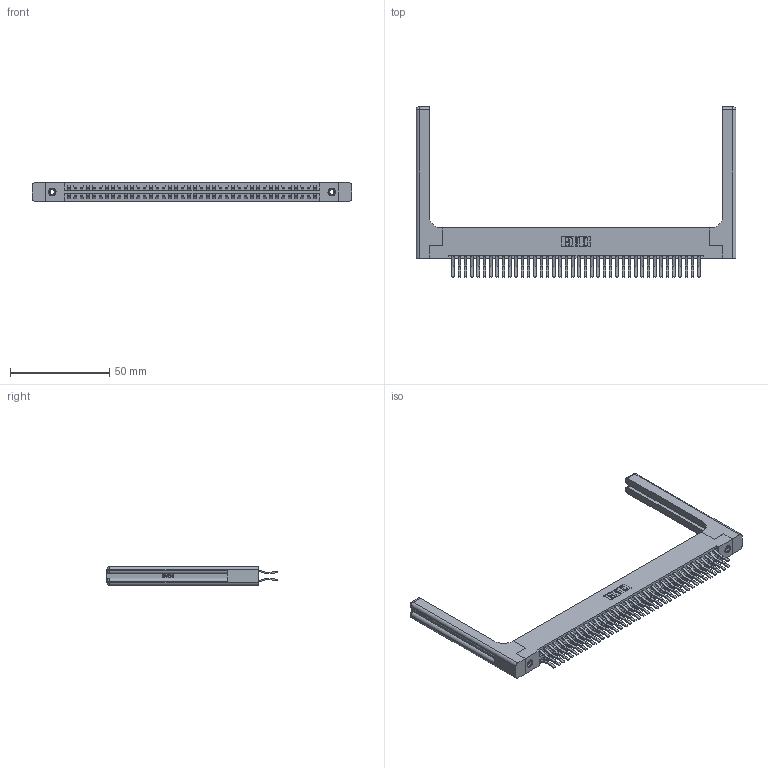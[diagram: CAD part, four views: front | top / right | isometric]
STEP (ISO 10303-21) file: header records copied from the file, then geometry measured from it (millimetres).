
FILE_DESCRIPTION (( 'STEP AP203' ), '1' );
FILE_NAME ('396-080-560-258.STEP', '2019-10-30T23:10:39', ( '' ), ( '' ), 'SwSTEP 2.0', 'SolidWorks 2016', '' );
FILE_SCHEMA (( 'CONFIG_CONTROL_DESIGN' ));
Length unit declared in the file: inch
Products named in the file (5): 345-250-001_345-250-001-102; 346-220-058_345-220-058; 396-080-560-258; 345-292-001_560 Tail; 346 Part_Flush Mounting Lugs - 0.156 Dia-TH
Assembly tree (85 placements, depth 2):
  396-080-560-258
    346 Part_Flush Mounting Lugs - 0.156 Dia-TH
    345-292-001_560 Tail  x80
    345-250-001_345-250-001-102  x2
    346-220-058_345-220-058  x2
Bounding box: 161.06 x 85.74 x 9.4 mm (x, y, z)
Volume: 23708.6 mm3; surface area: 28628 mm2
Topology: 85 solids, 85 shells, 4698 faces, 13875 edges, 9122 vertices
Faces by surface type: plane 3024, cylinder 1614, bspline 36, cone 12, sphere 8, torus 4
Entity records: 31644 total; most frequent: CARTESIAN_POINT 6225, ORIENTED_EDGE 4956, DIRECTION 4474, EDGE_CURVE 2478, LINE 2090, VECTOR 2090, VERTEX_POINT 1642, AXIS2_PLACEMENT_3D 1192
